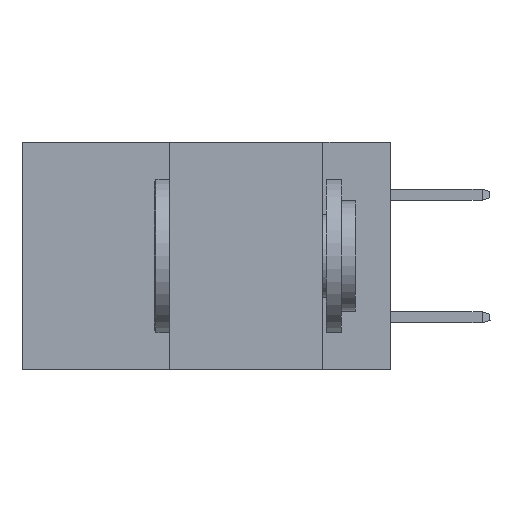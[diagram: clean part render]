
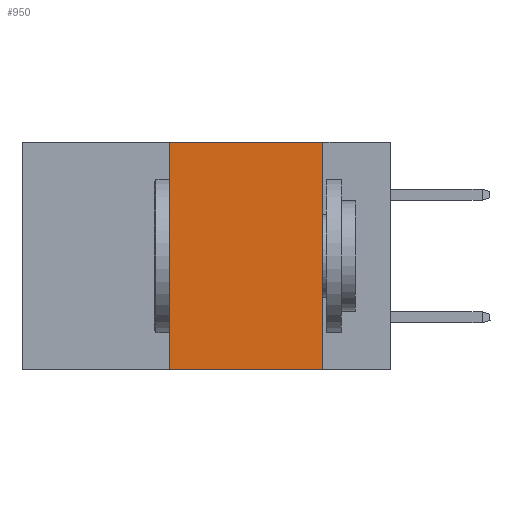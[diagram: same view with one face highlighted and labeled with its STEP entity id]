
A CAD part, left-side view. The second image highlights one B-rep face of the part: STEP entity #950.
In plain terms, the highlighted planar face has unit normal (-1, 0, 0).
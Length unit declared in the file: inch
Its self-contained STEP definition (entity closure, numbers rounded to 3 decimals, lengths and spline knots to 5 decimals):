
#15 = LINE ( 'NONE', #29093, #13497 ) ;
#822 = CARTESIAN_POINT ( 'NONE',  ( 0., 0.36, -0.37 ) ) ;
#950 = ADVANCED_FACE ( 'NONE', ( #2576 ), #28746, .F. ) ;
#1317 = DIRECTION ( 'NONE',  ( 0., 0., 1. ) ) ;
#1532 = CARTESIAN_POINT ( 'NONE',  ( 0., 0.6, -0.37 ) ) ;
#1588 = CARTESIAN_POINT ( 'NONE',  ( 0., 0.6, 0. ) ) ;
#1698 = CARTESIAN_POINT ( 'NONE',  ( 0., 0.6, 0. ) ) ;
#2406 = EDGE_LOOP ( 'NONE', ( #9493, #18962, #8102, #27045 ) ) ;
#2576 = FACE_OUTER_BOUND ( 'NONE', #2406, .T. ) ;
#3460 = VECTOR ( 'NONE', #12587, 39.37008 ) ;
#6469 = VECTOR ( 'NONE', #1317, 39.37008 ) ;
#7870 = VERTEX_POINT ( 'NONE', #822 ) ;
#7930 = LINE ( 'NONE', #26161, #6469 ) ;
#8102 = ORIENTED_EDGE ( 'NONE', *, *, #17662, .F. ) ;
#8583 = DIRECTION ( 'NONE',  ( 0., 0., -1. ) ) ;
#8887 = CARTESIAN_POINT ( 'NONE',  ( 0., 0.11, -0.37 ) ) ;
#9493 = ORIENTED_EDGE ( 'NONE', *, *, #23283, .F. ) ;
#10238 = LINE ( 'NONE', #1588, #3460 ) ;
#11170 = AXIS2_PLACEMENT_3D ( 'NONE', #1698, #24527, #8583 ) ;
#12587 = DIRECTION ( 'NONE',  ( 0., -1., 0. ) ) ;
#12847 = EDGE_CURVE ( 'NONE', #7870, #17907, #23142, .T. ) ;
#13497 = VECTOR ( 'NONE', #20130, 39.37008 ) ;
#17322 = DIRECTION ( 'NONE',  ( 0., -1., 0. ) ) ;
#17483 = VECTOR ( 'NONE', #17322, 39.37008 ) ;
#17662 = EDGE_CURVE ( 'NONE', #7870, #19292, #7930, .T. ) ;
#17907 = VERTEX_POINT ( 'NONE', #8887 ) ;
#18962 = ORIENTED_EDGE ( 'NONE', *, *, #20921, .F. ) ;
#19292 = VERTEX_POINT ( 'NONE', #23102 ) ;
#20130 = DIRECTION ( 'NONE',  ( 0., 0., -1. ) ) ;
#20921 = EDGE_CURVE ( 'NONE', #19292, #21024, #10238, .T. ) ;
#21024 = VERTEX_POINT ( 'NONE', #24520 ) ;
#23102 = CARTESIAN_POINT ( 'NONE',  ( 0., 0.36, 0. ) ) ;
#23142 = LINE ( 'NONE', #1532, #17483 ) ;
#23283 = EDGE_CURVE ( 'NONE', #21024, #17907, #15, .T. ) ;
#24520 = CARTESIAN_POINT ( 'NONE',  ( 0., 0.11, 0. ) ) ;
#24527 = DIRECTION ( 'NONE',  ( 1., 0., 0. ) ) ;
#26161 = CARTESIAN_POINT ( 'NONE',  ( 0., 0.36, 0. ) ) ;
#27045 = ORIENTED_EDGE ( 'NONE', *, *, #12847, .T. ) ;
#28746 = PLANE ( 'NONE',  #11170 ) ;
#29093 = CARTESIAN_POINT ( 'NONE',  ( 0., 0.11, 0. ) ) ;
